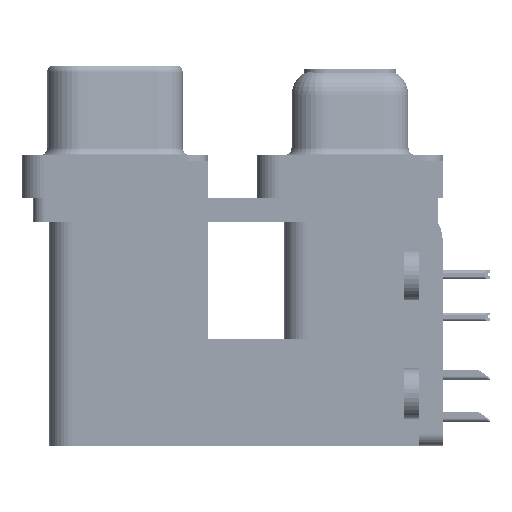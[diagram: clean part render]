
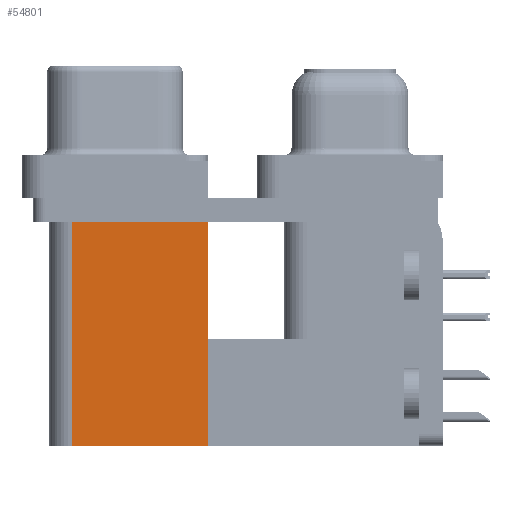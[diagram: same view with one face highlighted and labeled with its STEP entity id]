
A CAD part, left-side view. The second image highlights one B-rep face of the part: STEP entity #54801.
In plain terms, the highlighted planar face has unit normal (-1, 0, 0).
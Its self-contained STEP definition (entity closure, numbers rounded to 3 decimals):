
#1424 = VERTEX_POINT ( 'NONE', #37511 ) ;
#2557 = CARTESIAN_POINT ( 'NONE',  ( 3.7, 9.6, -19.2 ) ) ;
#2834 = CARTESIAN_POINT ( 'NONE',  ( 3.7, 18.8, -19.2 ) ) ;
#5119 = ORIENTED_EDGE ( 'NONE', *, *, #9460, .T. ) ;
#7995 = DIRECTION ( 'NONE',  ( 0., 1., 0. ) ) ;
#9460 = EDGE_CURVE ( 'NONE', #48817, #36446, #32655, .T. ) ;
#10140 = EDGE_CURVE ( 'NONE', #35965, #36446, #29310, .T. ) ;
#10249 = VECTOR ( 'NONE', #7995, 1000. ) ;
#13342 = CARTESIAN_POINT ( 'NONE',  ( 3.7, 18.8, -2.5 ) ) ;
#13787 = ORIENTED_EDGE ( 'NONE', *, *, #10140, .F. ) ;
#17801 = ORIENTED_EDGE ( 'NONE', *, *, #35998, .F. ) ;
#19878 = DIRECTION ( 'NONE',  ( 0., 1., 0. ) ) ;
#20406 = CARTESIAN_POINT ( 'NONE',  ( 3.7, 9.6, -2.5 ) ) ;
#21562 = ORIENTED_EDGE ( 'NONE', *, *, #25698, .T. ) ;
#25176 = DIRECTION ( 'NONE',  ( 0., 0., 1. ) ) ;
#25698 = EDGE_CURVE ( 'NONE', #1424, #48817, #50465, .T. ) ;
#29108 = LINE ( 'NONE', #2557, #10249 ) ;
#29310 = LINE ( 'NONE', #41833, #34568 ) ;
#30802 = VECTOR ( 'NONE', #25176, 1000. ) ;
#32655 = LINE ( 'NONE', #45180, #37139 ) ;
#32761 = FACE_OUTER_BOUND ( 'NONE', #36533, .T. ) ;
#34568 = VECTOR ( 'NONE', #50436, 1000. ) ;
#35965 = VERTEX_POINT ( 'NONE', #2834 ) ;
#35998 = EDGE_CURVE ( 'NONE', #1424, #35965, #29108, .T. ) ;
#36446 = VERTEX_POINT ( 'NONE', #13342 ) ;
#36533 = EDGE_LOOP ( 'NONE', ( #5119, #13787, #17801, #21562 ) ) ;
#37139 = VECTOR ( 'NONE', #19878, 1000. ) ;
#37460 = PLANE ( 'NONE',  #41102 ) ;
#37511 = CARTESIAN_POINT ( 'NONE',  ( 3.7, 9.6, -19.2 ) ) ;
#41102 = AXIS2_PLACEMENT_3D ( 'NONE', #53879, #49714, #41931 ) ;
#41833 = CARTESIAN_POINT ( 'NONE',  ( 3.7, 18.8, -19.2 ) ) ;
#41931 = DIRECTION ( 'NONE',  ( 0., 0., -1. ) ) ;
#45180 = CARTESIAN_POINT ( 'NONE',  ( 3.7, 9.6, -2.5 ) ) ;
#48817 = VERTEX_POINT ( 'NONE', #20406 ) ;
#49714 = DIRECTION ( 'NONE',  ( 1., 0., 0. ) ) ;
#50436 = DIRECTION ( 'NONE',  ( 0., 0., 1. ) ) ;
#50465 = LINE ( 'NONE', #54904, #30802 ) ;
#53879 = CARTESIAN_POINT ( 'NONE',  ( 3.7, 9.6, -19.2 ) ) ;
#54801 = ADVANCED_FACE ( 'NONE', ( #32761 ), #37460, .F. ) ;
#54904 = CARTESIAN_POINT ( 'NONE',  ( 3.7, 9.6, -19.2 ) ) ;
